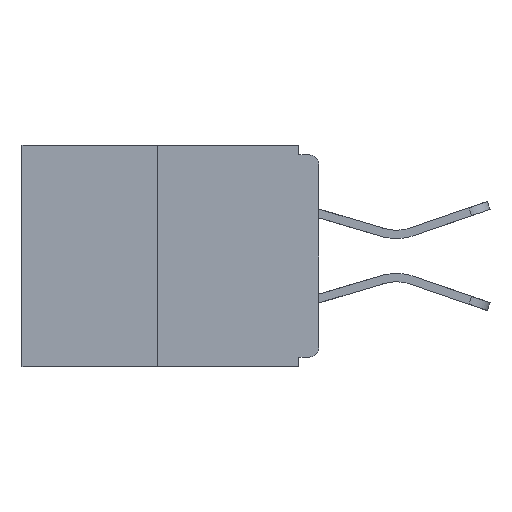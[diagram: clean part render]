
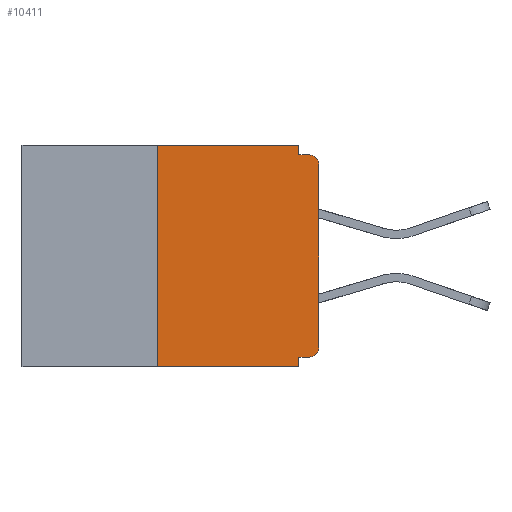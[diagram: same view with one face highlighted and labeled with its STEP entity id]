
A CAD part, left-side view. The second image highlights one B-rep face of the part: STEP entity #10411.
In plain terms, the highlighted planar face has unit normal (-1, 0, 0).
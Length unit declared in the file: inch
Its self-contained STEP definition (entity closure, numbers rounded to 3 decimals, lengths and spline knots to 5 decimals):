
#159 = DIRECTION ( 'NONE',  ( 1., 0., 0. ) ) ;
#397 = EDGE_CURVE ( 'NONE', #21717, #18239, #15263, .T. ) ;
#634 = LINE ( 'NONE', #24049, #4622 ) ;
#749 = DIRECTION ( 'NONE',  ( 0., 1., 0. ) ) ;
#992 = ORIENTED_EDGE ( 'NONE', *, *, #17286, .T. ) ;
#1259 = ORIENTED_EDGE ( 'NONE', *, *, #24989, .F. ) ;
#1548 = ORIENTED_EDGE ( 'NONE', *, *, #19430, .T. ) ;
#2039 = CIRCLE ( 'NONE', #21264, 0.015 ) ;
#2133 = EDGE_CURVE ( 'NONE', #17079, #21717, #18220, .T. ) ;
#2229 = EDGE_CURVE ( 'NONE', #12649, #17079, #19112, .T. ) ;
#2234 = DIRECTION ( 'NONE',  ( 0., 0., -1. ) ) ;
#2274 = CARTESIAN_POINT ( 'NONE',  ( 0., 0.25, 0. ) ) ;
#2399 = CARTESIAN_POINT ( 'NONE',  ( 0., 0.031, -0.343 ) ) ;
#3475 = ORIENTED_EDGE ( 'NONE', *, *, #7514, .F. ) ;
#3601 = DIRECTION ( 'NONE',  ( -1., 0., 0. ) ) ;
#4107 = DIRECTION ( 'NONE',  ( 0., 0., -1. ) ) ;
#4132 = CARTESIAN_POINT ( 'NONE',  ( 0., 0.031, -0.015 ) ) ;
#4138 = EDGE_LOOP ( 'NONE', ( #17374, #9003, #992, #10695, #1259, #25099, #1548, #18893, #3475, #6353 ) ) ;
#4216 = AXIS2_PLACEMENT_3D ( 'NONE', #19648, #11925, #15654 ) ;
#4622 = VECTOR ( 'NONE', #749, 39.37008 ) ;
#4987 = LINE ( 'NONE', #2399, #23543 ) ;
#5064 = DIRECTION ( 'NONE',  ( 0., -1., 0. ) ) ;
#5861 = CARTESIAN_POINT ( 'NONE',  ( 0., 0., -0.313 ) ) ;
#6224 = CARTESIAN_POINT ( 'NONE',  ( 0., 0.031, -0.343 ) ) ;
#6353 = ORIENTED_EDGE ( 'NONE', *, *, #397, .F. ) ;
#6390 = EDGE_CURVE ( 'NONE', #11323, #24562, #12547, .T. ) ;
#6790 = VERTEX_POINT ( 'NONE', #20180 ) ;
#7080 = CARTESIAN_POINT ( 'NONE',  ( 0., 0., -0.015 ) ) ;
#7514 = EDGE_CURVE ( 'NONE', #18239, #15913, #14563, .T. ) ;
#7712 = CARTESIAN_POINT ( 'NONE',  ( 0., 0.015, -0.328 ) ) ;
#8033 = CARTESIAN_POINT ( 'NONE',  ( 0., 0.25, -0.343 ) ) ;
#8794 = VECTOR ( 'NONE', #17995, 39.37008 ) ;
#9003 = ORIENTED_EDGE ( 'NONE', *, *, #2229, .F. ) ;
#10411 = ADVANCED_FACE ( 'NONE', ( #18230 ), #17708, .F. ) ;
#10571 = VERTEX_POINT ( 'NONE', #6224 ) ;
#10695 = ORIENTED_EDGE ( 'NONE', *, *, #23509, .F. ) ;
#10815 = AXIS2_PLACEMENT_3D ( 'NONE', #23293, #159, #4107 ) ;
#11177 = DIRECTION ( 'NONE',  ( 0., -1., 0. ) ) ;
#11323 = VERTEX_POINT ( 'NONE', #7712 ) ;
#11460 = CARTESIAN_POINT ( 'NONE',  ( 0., 0.46, 0. ) ) ;
#11788 = LINE ( 'NONE', #14751, #15109 ) ;
#11925 = DIRECTION ( 'NONE',  ( -1., 0., 0. ) ) ;
#12547 = CIRCLE ( 'NONE', #4216, 0.015 ) ;
#12649 = VERTEX_POINT ( 'NONE', #8033 ) ;
#13418 = DIRECTION ( 'NONE',  ( 0., -1., 0. ) ) ;
#13654 = DIRECTION ( 'NONE',  ( 0., 0., 1. ) ) ;
#14563 = LINE ( 'NONE', #7080, #23999 ) ;
#14650 = VECTOR ( 'NONE', #25129, 39.37008 ) ;
#14698 = LINE ( 'NONE', #15791, #22897 ) ;
#14751 = CARTESIAN_POINT ( 'NONE',  ( 0., 0.46, -0.343 ) ) ;
#15109 = VECTOR ( 'NONE', #11177, 39.37008 ) ;
#15263 = LINE ( 'NONE', #19570, #14650 ) ;
#15654 = DIRECTION ( 'NONE',  ( 0., 0., -1. ) ) ;
#15791 = CARTESIAN_POINT ( 'NONE',  ( 0., 0., 0. ) ) ;
#15913 = VERTEX_POINT ( 'NONE', #21970 ) ;
#15937 = CARTESIAN_POINT ( 'NONE',  ( 0., 0.031, -0.328 ) ) ;
#17079 = VERTEX_POINT ( 'NONE', #17257 ) ;
#17257 = CARTESIAN_POINT ( 'NONE',  ( 0., 0.25, 0. ) ) ;
#17286 = EDGE_CURVE ( 'NONE', #12649, #10571, #11788, .T. ) ;
#17355 = EDGE_CURVE ( 'NONE', #6790, #15913, #2039, .T. ) ;
#17374 = ORIENTED_EDGE ( 'NONE', *, *, #2133, .F. ) ;
#17708 = PLANE ( 'NONE',  #10815 ) ;
#17995 = DIRECTION ( 'NONE',  ( 0., 0., 1. ) ) ;
#18220 = LINE ( 'NONE', #11460, #22752 ) ;
#18230 = FACE_OUTER_BOUND ( 'NONE', #4138, .T. ) ;
#18239 = VERTEX_POINT ( 'NONE', #4132 ) ;
#18893 = ORIENTED_EDGE ( 'NONE', *, *, #17355, .T. ) ;
#19011 = VERTEX_POINT ( 'NONE', #15937 ) ;
#19112 = LINE ( 'NONE', #2274, #8794 ) ;
#19430 = EDGE_CURVE ( 'NONE', #24562, #6790, #14698, .T. ) ;
#19570 = CARTESIAN_POINT ( 'NONE',  ( 0., 0.031, 0. ) ) ;
#19648 = CARTESIAN_POINT ( 'NONE',  ( 0., 0.015, -0.313 ) ) ;
#20180 = CARTESIAN_POINT ( 'NONE',  ( 0., 0., -0.03 ) ) ;
#21264 = AXIS2_PLACEMENT_3D ( 'NONE', #24802, #3601, #22795 ) ;
#21717 = VERTEX_POINT ( 'NONE', #24070 ) ;
#21970 = CARTESIAN_POINT ( 'NONE',  ( 0., 0.015, -0.015 ) ) ;
#22752 = VECTOR ( 'NONE', #13418, 39.37008 ) ;
#22795 = DIRECTION ( 'NONE',  ( 0., 0., -1. ) ) ;
#22897 = VECTOR ( 'NONE', #13654, 39.37008 ) ;
#23293 = CARTESIAN_POINT ( 'NONE',  ( 0., 0.46, 0. ) ) ;
#23509 = EDGE_CURVE ( 'NONE', #19011, #10571, #4987, .T. ) ;
#23543 = VECTOR ( 'NONE', #2234, 39.37008 ) ;
#23999 = VECTOR ( 'NONE', #5064, 39.37008 ) ;
#24049 = CARTESIAN_POINT ( 'NONE',  ( 0., 0., -0.328 ) ) ;
#24070 = CARTESIAN_POINT ( 'NONE',  ( 0., 0.031, 0. ) ) ;
#24562 = VERTEX_POINT ( 'NONE', #5861 ) ;
#24802 = CARTESIAN_POINT ( 'NONE',  ( 0., 0.015, -0.03 ) ) ;
#24989 = EDGE_CURVE ( 'NONE', #11323, #19011, #634, .T. ) ;
#25099 = ORIENTED_EDGE ( 'NONE', *, *, #6390, .T. ) ;
#25129 = DIRECTION ( 'NONE',  ( 0., 0., -1. ) ) ;
